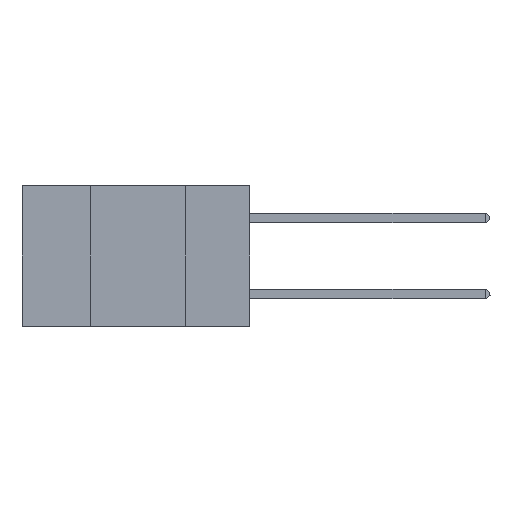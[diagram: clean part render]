
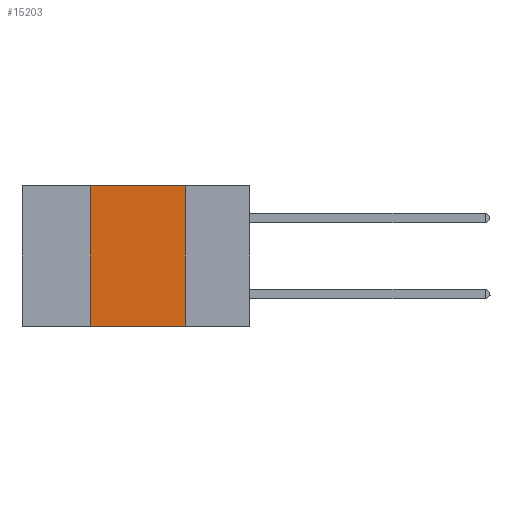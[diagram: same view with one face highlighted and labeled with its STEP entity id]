
A CAD part, left-side view. The second image highlights one B-rep face of the part: STEP entity #15203.
In plain terms, the highlighted planar face has unit normal (-1, 0, 0).
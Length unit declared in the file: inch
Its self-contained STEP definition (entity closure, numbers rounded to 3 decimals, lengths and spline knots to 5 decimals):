
#142 = LINE ( 'NONE', #20777, #24357 ) ;
#207 = VERTEX_POINT ( 'NONE', #20173 ) ;
#665 = FACE_OUTER_BOUND ( 'NONE', #2738, .T. ) ;
#1753 = EDGE_CURVE ( 'NONE', #22006, #4616, #14310, .T. ) ;
#2738 = EDGE_LOOP ( 'NONE', ( #10350, #2855, #6235, #4181 ) ) ;
#2776 = CARTESIAN_POINT ( 'NONE',  ( 0., 0.6, 0. ) ) ;
#2855 = ORIENTED_EDGE ( 'NONE', *, *, #10650, .F. ) ;
#4170 = CARTESIAN_POINT ( 'NONE',  ( 0., 0.42, 0. ) ) ;
#4181 = ORIENTED_EDGE ( 'NONE', *, *, #17551, .T. ) ;
#4616 = VERTEX_POINT ( 'NONE', #7558 ) ;
#6235 = ORIENTED_EDGE ( 'NONE', *, *, #22213, .F. ) ;
#6407 = DIRECTION ( 'NONE',  ( 0., 0., -1. ) ) ;
#7558 = CARTESIAN_POINT ( 'NONE',  ( 0., 0.17, -0.37 ) ) ;
#10350 = ORIENTED_EDGE ( 'NONE', *, *, #1753, .F. ) ;
#10650 = EDGE_CURVE ( 'NONE', #207, #22006, #23018, .T. ) ;
#12180 = DIRECTION ( 'NONE',  ( 0., -1., 0. ) ) ;
#13092 = PLANE ( 'NONE',  #14081 ) ;
#14081 = AXIS2_PLACEMENT_3D ( 'NONE', #19578, #23918, #6407 ) ;
#14113 = DIRECTION ( 'NONE',  ( 0., -1., 0. ) ) ;
#14310 = LINE ( 'NONE', #19121, #22069 ) ;
#14629 = LINE ( 'NONE', #4170, #16657 ) ;
#14685 = DIRECTION ( 'NONE',  ( 0., 0., -1. ) ) ;
#15203 = ADVANCED_FACE ( 'NONE', ( #665 ), #13092, .F. ) ;
#16657 = VECTOR ( 'NONE', #25516, 39.37008 ) ;
#17551 = EDGE_CURVE ( 'NONE', #19541, #4616, #142, .T. ) ;
#18398 = CARTESIAN_POINT ( 'NONE',  ( 0., 0.42, -0.37 ) ) ;
#19012 = VECTOR ( 'NONE', #14113, 39.37008 ) ;
#19121 = CARTESIAN_POINT ( 'NONE',  ( 0., 0.17, 0. ) ) ;
#19541 = VERTEX_POINT ( 'NONE', #18398 ) ;
#19578 = CARTESIAN_POINT ( 'NONE',  ( 0., 0.6, 0. ) ) ;
#20173 = CARTESIAN_POINT ( 'NONE',  ( 0., 0.42, 0. ) ) ;
#20777 = CARTESIAN_POINT ( 'NONE',  ( 0., 0.6, -0.37 ) ) ;
#22006 = VERTEX_POINT ( 'NONE', #26931 ) ;
#22069 = VECTOR ( 'NONE', #14685, 39.37008 ) ;
#22213 = EDGE_CURVE ( 'NONE', #19541, #207, #14629, .T. ) ;
#23018 = LINE ( 'NONE', #2776, #19012 ) ;
#23918 = DIRECTION ( 'NONE',  ( 1., 0., 0. ) ) ;
#24357 = VECTOR ( 'NONE', #12180, 39.37008 ) ;
#25516 = DIRECTION ( 'NONE',  ( 0., 0., 1. ) ) ;
#26931 = CARTESIAN_POINT ( 'NONE',  ( 0., 0.17, 0. ) ) ;
